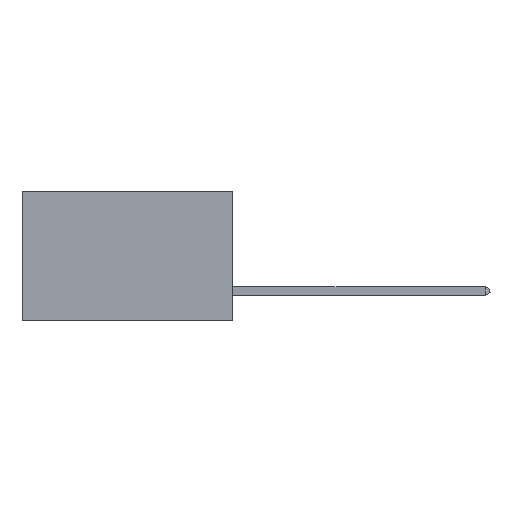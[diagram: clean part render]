
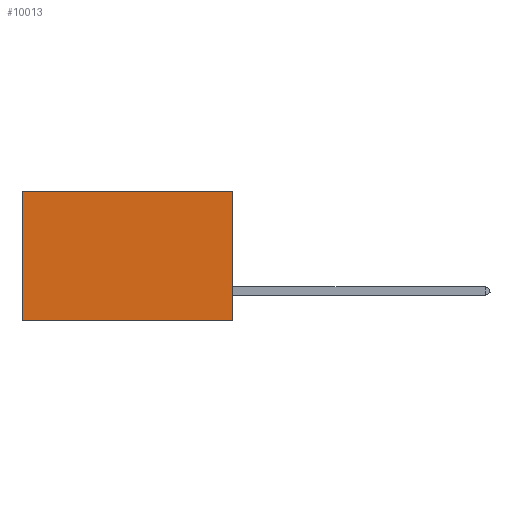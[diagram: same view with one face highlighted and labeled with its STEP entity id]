
A CAD part, left-side view. The second image highlights one B-rep face of the part: STEP entity #10013.
In plain terms, the highlighted planar face has unit normal (-1, 0, 0).
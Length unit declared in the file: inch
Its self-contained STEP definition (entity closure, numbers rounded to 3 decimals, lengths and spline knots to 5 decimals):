
#615 = ORIENTED_EDGE ( 'NONE', *, *, #3843, .T. ) ;
#837 = EDGE_CURVE ( 'NONE', #13844, #9185, #17745, .T. ) ;
#3620 = ORIENTED_EDGE ( 'NONE', *, *, #15528, .F. ) ;
#3654 = VECTOR ( 'NONE', #6254, 39.37008 ) ;
#3843 = EDGE_CURVE ( 'NONE', #18499, #13844, #6203, .T. ) ;
#5000 = AXIS2_PLACEMENT_3D ( 'NONE', #18719, #9823, #22318 ) ;
#5847 = LINE ( 'NONE', #11530, #3654 ) ;
#6203 = LINE ( 'NONE', #7752, #8453 ) ;
#6235 = PLANE ( 'NONE',  #5000 ) ;
#6254 = DIRECTION ( 'NONE',  ( 0., 0., -1. ) ) ;
#6312 = DIRECTION ( 'NONE',  ( 0., 0., -1. ) ) ;
#6445 = VERTEX_POINT ( 'NONE', #18808 ) ;
#7556 = ORIENTED_EDGE ( 'NONE', *, *, #837, .T. ) ;
#7752 = CARTESIAN_POINT ( 'NONE',  ( 0.2875, 0., 0. ) ) ;
#8453 = VECTOR ( 'NONE', #21334, 39.37008 ) ;
#9185 = VERTEX_POINT ( 'NONE', #11923 ) ;
#9596 = CARTESIAN_POINT ( 'NONE',  ( 0.2875, 0., -0.37 ) ) ;
#9823 = DIRECTION ( 'NONE',  ( 1., 0., 0. ) ) ;
#10013 = ADVANCED_FACE ( 'NONE', ( #18061 ), #6235, .F. ) ;
#11113 = EDGE_CURVE ( 'NONE', #6445, #9185, #12679, .T. ) ;
#11530 = CARTESIAN_POINT ( 'NONE',  ( 0.2875, 0., 0. ) ) ;
#11923 = CARTESIAN_POINT ( 'NONE',  ( 0.2875, 0.6, -0.37 ) ) ;
#12679 = LINE ( 'NONE', #9596, #12946 ) ;
#12946 = VECTOR ( 'NONE', #18256, 39.37008 ) ;
#13537 = VECTOR ( 'NONE', #6312, 39.37008 ) ;
#13844 = VERTEX_POINT ( 'NONE', #19058 ) ;
#15528 = EDGE_CURVE ( 'NONE', #18499, #6445, #5847, .T. ) ;
#15537 = CARTESIAN_POINT ( 'NONE',  ( 0.2875, 0., 0. ) ) ;
#15933 = EDGE_LOOP ( 'NONE', ( #7556, #18360, #3620, #615 ) ) ;
#17745 = LINE ( 'NONE', #20586, #13537 ) ;
#18061 = FACE_OUTER_BOUND ( 'NONE', #15933, .T. ) ;
#18256 = DIRECTION ( 'NONE',  ( 0., 1., 0. ) ) ;
#18360 = ORIENTED_EDGE ( 'NONE', *, *, #11113, .F. ) ;
#18499 = VERTEX_POINT ( 'NONE', #15537 ) ;
#18719 = CARTESIAN_POINT ( 'NONE',  ( 0.2875, 0., 0. ) ) ;
#18808 = CARTESIAN_POINT ( 'NONE',  ( 0.2875, 0., -0.37 ) ) ;
#19058 = CARTESIAN_POINT ( 'NONE',  ( 0.2875, 0.6, 0. ) ) ;
#20586 = CARTESIAN_POINT ( 'NONE',  ( 0.2875, 0.6, 0. ) ) ;
#21334 = DIRECTION ( 'NONE',  ( 0., 1., 0. ) ) ;
#22318 = DIRECTION ( 'NONE',  ( 0., 0., -1. ) ) ;
